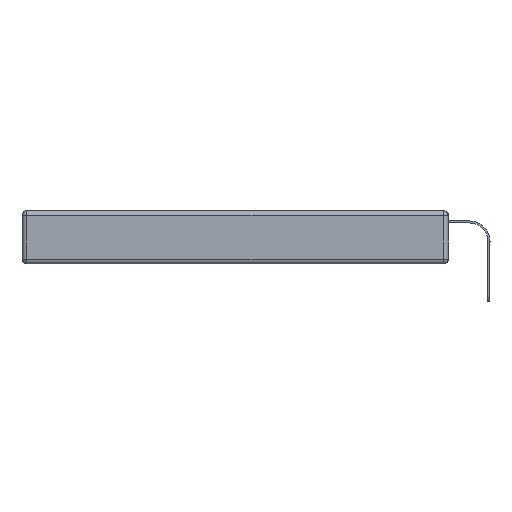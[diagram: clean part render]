
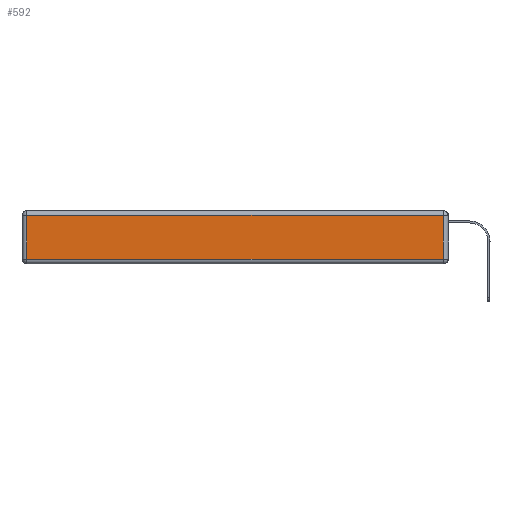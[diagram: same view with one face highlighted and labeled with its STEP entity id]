
A CAD part, left-side view. The second image highlights one B-rep face of the part: STEP entity #592.
In plain terms, the highlighted planar face has unit normal (-1, 0, 0).
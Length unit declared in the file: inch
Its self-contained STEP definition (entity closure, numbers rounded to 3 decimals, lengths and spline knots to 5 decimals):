
#224 = VECTOR ( 'NONE', #11359, 39.37008 ) ;
#592 = ADVANCED_FACE ( 'NONE', ( #12263 ), #3714, .T. ) ;
#600 = EDGE_LOOP ( 'NONE', ( #3669, #3633, #1662, #13750 ) ) ;
#783 = CARTESIAN_POINT ( 'NONE',  ( 0., 2.72, -0.343 ) ) ;
#1383 = DIRECTION ( 'NONE',  ( 0., 0., 1. ) ) ;
#1662 = ORIENTED_EDGE ( 'NONE', *, *, #11000, .T. ) ;
#2183 = LINE ( 'NONE', #14079, #7781 ) ;
#2256 = CARTESIAN_POINT ( 'NONE',  ( 0., 0.03, -0.343 ) ) ;
#3361 = VERTEX_POINT ( 'NONE', #8785 ) ;
#3425 = DIRECTION ( 'NONE',  ( 0., -1., 0. ) ) ;
#3633 = ORIENTED_EDGE ( 'NONE', *, *, #6806, .T. ) ;
#3669 = ORIENTED_EDGE ( 'NONE', *, *, #10720, .T. ) ;
#3714 = PLANE ( 'NONE',  #6684 ) ;
#3734 = CARTESIAN_POINT ( 'NONE',  ( 0., 0.03, -0.313 ) ) ;
#5048 = VERTEX_POINT ( 'NONE', #3734 ) ;
#6684 = AXIS2_PLACEMENT_3D ( 'NONE', #13511, #8447, #1383 ) ;
#6806 = EDGE_CURVE ( 'NONE', #5048, #14773, #10643, .T. ) ;
#7302 = VECTOR ( 'NONE', #9473, 39.37008 ) ;
#7781 = VECTOR ( 'NONE', #3425, 39.37008 ) ;
#7836 = EDGE_CURVE ( 'NONE', #3361, #9574, #14946, .T. ) ;
#8447 = DIRECTION ( 'NONE',  ( -1., 0., 0. ) ) ;
#8774 = CARTESIAN_POINT ( 'NONE',  ( 0., 2.75, -0.03 ) ) ;
#8785 = CARTESIAN_POINT ( 'NONE',  ( 0., 2.72, -0.03 ) ) ;
#8817 = CARTESIAN_POINT ( 'NONE',  ( 0., 0.03, -0.03 ) ) ;
#9473 = DIRECTION ( 'NONE',  ( 0., 0., 1. ) ) ;
#9574 = VERTEX_POINT ( 'NONE', #13581 ) ;
#10643 = LINE ( 'NONE', #2256, #7302 ) ;
#10720 = EDGE_CURVE ( 'NONE', #9574, #5048, #2183, .T. ) ;
#11000 = EDGE_CURVE ( 'NONE', #14773, #3361, #12436, .T. ) ;
#11359 = DIRECTION ( 'NONE',  ( 0., 0., -1. ) ) ;
#12263 = FACE_OUTER_BOUND ( 'NONE', #600, .T. ) ;
#12436 = LINE ( 'NONE', #8774, #13528 ) ;
#13511 = CARTESIAN_POINT ( 'NONE',  ( 0., 0., -0.343 ) ) ;
#13528 = VECTOR ( 'NONE', #13754, 39.37008 ) ;
#13581 = CARTESIAN_POINT ( 'NONE',  ( 0., 2.72, -0.313 ) ) ;
#13750 = ORIENTED_EDGE ( 'NONE', *, *, #7836, .T. ) ;
#13754 = DIRECTION ( 'NONE',  ( 0., 1., 0. ) ) ;
#14079 = CARTESIAN_POINT ( 'NONE',  ( 0., 0., -0.313 ) ) ;
#14773 = VERTEX_POINT ( 'NONE', #8817 ) ;
#14946 = LINE ( 'NONE', #783, #224 ) ;
